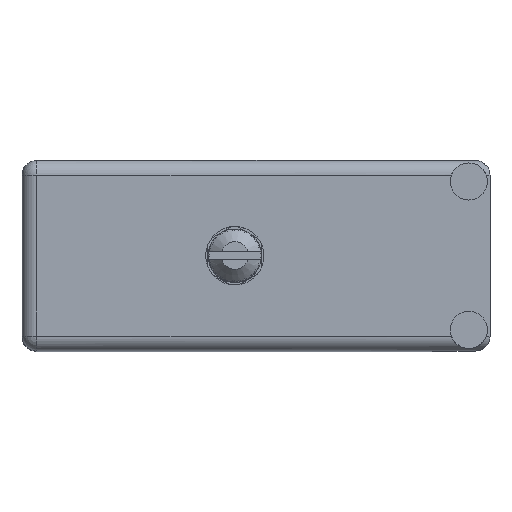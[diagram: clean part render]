
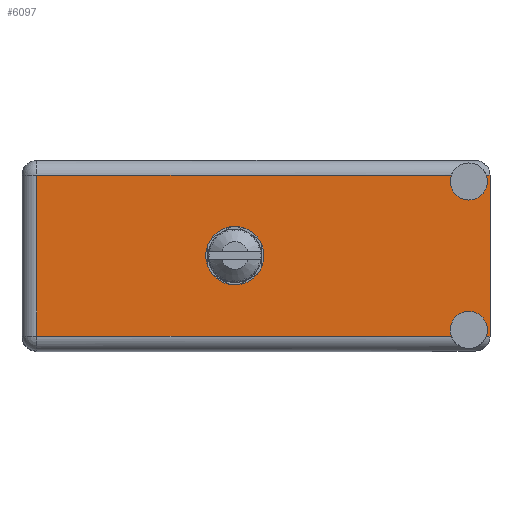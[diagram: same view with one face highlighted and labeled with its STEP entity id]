
A CAD part, top view. The second image highlights one B-rep face of the part: STEP entity #6097.
In plain terms, the highlighted face is planar.
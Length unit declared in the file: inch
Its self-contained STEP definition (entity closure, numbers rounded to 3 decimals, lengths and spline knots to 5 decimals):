
#940 = CIRCLE ( 'NONE', #45703, 0.0875 ) ;
#1325 = AXIS2_PLACEMENT_3D ( 'NONE', #93922, #35414, #45657 ) ;
#1718 = CARTESIAN_POINT ( 'NONE',  ( 2.108, 1.566, -0.7995 ) ) ;
#2294 = ORIENTED_EDGE ( 'NONE', *, *, #59275, .F. ) ;
#4606 = DIRECTION ( 'NONE',  ( 0., 0., 1. ) ) ;
#5187 = ORIENTED_EDGE ( 'NONE', *, *, #101737, .F. ) ;
#6097 = ADVANCED_FACE ( 'NONE', ( #33491, #54830 ), #50393, .T. ) ;
#6137 = VERTEX_POINT ( 'NONE', #101793 ) ;
#7043 = LINE ( 'NONE', #60360, #47409 ) ;
#8255 = ORIENTED_EDGE ( 'NONE', *, *, #10665, .T. ) ;
#9894 = DIRECTION ( 'NONE',  ( 0., 1., 0. ) ) ;
#10665 = EDGE_CURVE ( 'NONE', #56563, #88810, #27906, .T. ) ;
#12514 = ORIENTED_EDGE ( 'NONE', *, *, #84109, .F. ) ;
#13126 = CARTESIAN_POINT ( 'NONE',  ( 2.108, 1.566, -0.187 ) ) ;
#13408 = CARTESIAN_POINT ( 'NONE',  ( 2.208, 1.566, 0. ) ) ;
#14129 = CARTESIAN_POINT ( 'NONE',  ( 2.108, 1.566, -0.7995 ) ) ;
#14239 = EDGE_CURVE ( 'NONE', #71143, #88810, #85445, .T. ) ;
#15464 = CARTESIAN_POINT ( 'NONE',  ( 1.004, 1.566, -0.312 ) ) ;
#15601 = CARTESIAN_POINT ( 'NONE',  ( 2.19038, 1.566, -0.07 ) ) ;
#15609 = CIRCLE ( 'NONE', #19954, 0.0875 ) ;
#16363 = ORIENTED_EDGE ( 'NONE', *, *, #21741, .T. ) ;
#19314 = AXIS2_PLACEMENT_3D ( 'NONE', #34601, #9894, #74418 ) ;
#19496 = VERTEX_POINT ( 'NONE', #90046 ) ;
#19882 = DIRECTION ( 'NONE',  ( 0., 0., 1. ) ) ;
#19954 = AXIS2_PLACEMENT_3D ( 'NONE', #14129, #77172, #4606 ) ;
#20211 = ORIENTED_EDGE ( 'NONE', *, *, #14239, .F. ) ;
#20507 = VERTEX_POINT ( 'NONE', #85977 ) ;
#20612 = LINE ( 'NONE', #31416, #89971 ) ;
#21741 = EDGE_CURVE ( 'NONE', #33353, #101649, #20612, .T. ) ;
#23265 = CIRCLE ( 'NONE', #19314, 0.1375 ) ;
#23577 = DIRECTION ( 'NONE',  ( -1., 0., 0. ) ) ;
#26574 = CARTESIAN_POINT ( 'NONE',  ( 1.004, 1.566, -0.4495 ) ) ;
#27906 = LINE ( 'NONE', #65889, #65705 ) ;
#29969 = LINE ( 'NONE', #42970, #79085 ) ;
#31416 = CARTESIAN_POINT ( 'NONE',  ( 0., 1.566, -0.829 ) ) ;
#33022 = DIRECTION ( 'NONE',  ( 0., 1., 0. ) ) ;
#33154 = DIRECTION ( 'NONE',  ( 0., 0., 1. ) ) ;
#33353 = VERTEX_POINT ( 'NONE', #73511 ) ;
#33491 = FACE_BOUND ( 'NONE', #73581, .T. ) ;
#33527 = VERTEX_POINT ( 'NONE', #49157 ) ;
#34601 = CARTESIAN_POINT ( 'NONE',  ( 1.004, 1.566, -0.4495 ) ) ;
#35174 = CIRCLE ( 'NONE', #51373, 0.0875 ) ;
#35221 = CARTESIAN_POINT ( 'NONE',  ( 0., 1.566, -0.899 ) ) ;
#35414 = DIRECTION ( 'NONE',  ( 0., 1., 0. ) ) ;
#36465 = ORIENTED_EDGE ( 'NONE', *, *, #98309, .F. ) ;
#37049 = EDGE_CURVE ( 'NONE', #43279, #71143, #940, .T. ) ;
#37577 = AXIS2_PLACEMENT_3D ( 'NONE', #35221, #91555, #43318 ) ;
#39632 = CARTESIAN_POINT ( 'NONE',  ( 2.19038, 1.566, -0.829 ) ) ;
#40418 = CARTESIAN_POINT ( 'NONE',  ( 2.108, 1.566, -0.0995 ) ) ;
#41566 = EDGE_CURVE ( 'NONE', #20507, #6137, #7043, .T. ) ;
#42641 = DIRECTION ( 'NONE',  ( 1., 0., 0. ) ) ;
#42970 = CARTESIAN_POINT ( 'NONE',  ( 2.208, 1.566, -0.07 ) ) ;
#43279 = VERTEX_POINT ( 'NONE', #15601 ) ;
#43318 = DIRECTION ( 'NONE',  ( 0., 0., 1. ) ) ;
#45657 = DIRECTION ( 'NONE',  ( 0., 0., 1. ) ) ;
#45703 = AXIS2_PLACEMENT_3D ( 'NONE', #40418, #33022, #97470 ) ;
#47409 = VECTOR ( 'NONE', #83275, 39.37008 ) ;
#48994 = ORIENTED_EDGE ( 'NONE', *, *, #37049, .F. ) ;
#49157 = CARTESIAN_POINT ( 'NONE',  ( 1.004, 1.566, -0.587 ) ) ;
#50393 = PLANE ( 'NONE',  #37577 ) ;
#51373 = AXIS2_PLACEMENT_3D ( 'NONE', #1718, #98574, #60443 ) ;
#51452 = CARTESIAN_POINT ( 'NONE',  ( 2.02562, 1.566, -0.07 ) ) ;
#52889 = DIRECTION ( 'NONE',  ( 0., 0., 1. ) ) ;
#53006 = VERTEX_POINT ( 'NONE', #15464 ) ;
#54830 = FACE_OUTER_BOUND ( 'NONE', #87986, .T. ) ;
#55526 = AXIS2_PLACEMENT_3D ( 'NONE', #26574, #82948, #19882 ) ;
#56563 = VERTEX_POINT ( 'NONE', #95766 ) ;
#57328 = CIRCLE ( 'NONE', #55526, 0.1375 ) ;
#59132 = ORIENTED_EDGE ( 'NONE', *, *, #101303, .F. ) ;
#59275 = EDGE_CURVE ( 'NONE', #60454, #101649, #35174, .T. ) ;
#60360 = CARTESIAN_POINT ( 'NONE',  ( 0., 1.566, -0.829 ) ) ;
#60443 = DIRECTION ( 'NONE',  ( 0., 0., 1. ) ) ;
#60454 = VERTEX_POINT ( 'NONE', #98729 ) ;
#60826 = EDGE_CURVE ( 'NONE', #43279, #19496, #29969, .T. ) ;
#65705 = VECTOR ( 'NONE', #42641, 39.37008 ) ;
#65889 = CARTESIAN_POINT ( 'NONE',  ( 2.208, 1.566, -0.07 ) ) ;
#67439 = EDGE_CURVE ( 'NONE', #6137, #56563, #77020, .T. ) ;
#67925 = VECTOR ( 'NONE', #52889, 39.37008 ) ;
#71143 = VERTEX_POINT ( 'NONE', #13126 ) ;
#72687 = ORIENTED_EDGE ( 'NONE', *, *, #67439, .T. ) ;
#73511 = CARTESIAN_POINT ( 'NONE',  ( 2.208, 1.566, -0.829 ) ) ;
#73531 = DIRECTION ( 'NONE',  ( 1., 0., 0. ) ) ;
#73581 = EDGE_LOOP ( 'NONE', ( #5187, #59132 ) ) ;
#74418 = DIRECTION ( 'NONE',  ( 0., 0., 1. ) ) ;
#77020 = LINE ( 'NONE', #80363, #83245 ) ;
#77172 = DIRECTION ( 'NONE',  ( 0., 1., 0. ) ) ;
#79085 = VECTOR ( 'NONE', #73531, 39.37008 ) ;
#80363 = CARTESIAN_POINT ( 'NONE',  ( 0.07, 1.566, -0.899 ) ) ;
#82948 = DIRECTION ( 'NONE',  ( 0., 1., 0. ) ) ;
#83245 = VECTOR ( 'NONE', #33154, 39.37008 ) ;
#83275 = DIRECTION ( 'NONE',  ( -1., 0., 0. ) ) ;
#84109 = EDGE_CURVE ( 'NONE', #20507, #60454, #15609, .T. ) ;
#85445 = CIRCLE ( 'NONE', #1325, 0.0875 ) ;
#85977 = CARTESIAN_POINT ( 'NONE',  ( 2.02562, 1.566, -0.829 ) ) ;
#87986 = EDGE_LOOP ( 'NONE', ( #8255, #20211, #48994, #98190, #36465, #16363, #2294, #12514, #90893, #72687 ) ) ;
#88810 = VERTEX_POINT ( 'NONE', #51452 ) ;
#89351 = LINE ( 'NONE', #13408, #67925 ) ;
#89971 = VECTOR ( 'NONE', #23577, 39.37008 ) ;
#90046 = CARTESIAN_POINT ( 'NONE',  ( 2.208, 1.566, -0.07 ) ) ;
#90893 = ORIENTED_EDGE ( 'NONE', *, *, #41566, .T. ) ;
#91555 = DIRECTION ( 'NONE',  ( 0., 1., 0. ) ) ;
#93922 = CARTESIAN_POINT ( 'NONE',  ( 2.108, 1.566, -0.0995 ) ) ;
#95766 = CARTESIAN_POINT ( 'NONE',  ( 0.07, 1.566, -0.07 ) ) ;
#97470 = DIRECTION ( 'NONE',  ( 0., 0., 1. ) ) ;
#98190 = ORIENTED_EDGE ( 'NONE', *, *, #60826, .T. ) ;
#98309 = EDGE_CURVE ( 'NONE', #33353, #19496, #89351, .T. ) ;
#98574 = DIRECTION ( 'NONE',  ( 0., 1., 0. ) ) ;
#98729 = CARTESIAN_POINT ( 'NONE',  ( 2.108, 1.566, -0.712 ) ) ;
#101303 = EDGE_CURVE ( 'NONE', #33527, #53006, #57328, .T. ) ;
#101649 = VERTEX_POINT ( 'NONE', #39632 ) ;
#101737 = EDGE_CURVE ( 'NONE', #53006, #33527, #23265, .T. ) ;
#101793 = CARTESIAN_POINT ( 'NONE',  ( 0.07, 1.566, -0.829 ) ) ;
